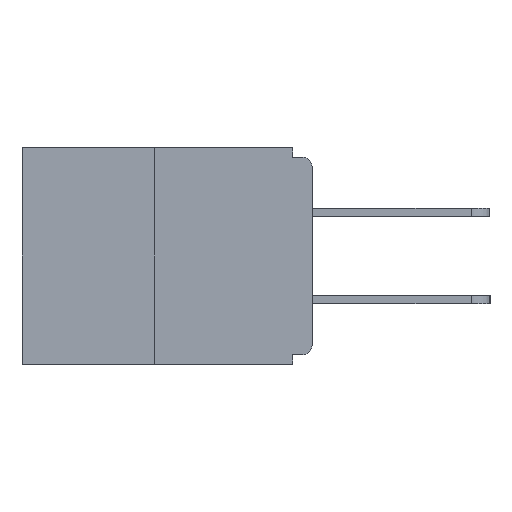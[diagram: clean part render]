
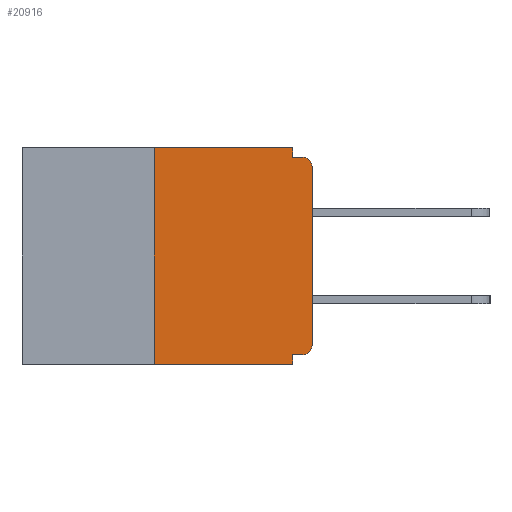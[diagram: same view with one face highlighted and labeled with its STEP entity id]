
A CAD part, left-side view. The second image highlights one B-rep face of the part: STEP entity #20916.
In plain terms, the highlighted planar face has unit normal (-1, 0, 0).
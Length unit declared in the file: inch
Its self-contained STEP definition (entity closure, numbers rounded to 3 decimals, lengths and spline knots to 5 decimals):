
#261 = CARTESIAN_POINT ( 'NONE',  ( 0., 0.015, -0.313 ) ) ;
#347 = EDGE_CURVE ( 'NONE', #24969, #27479, #17518, .T. ) ;
#1140 = VERTEX_POINT ( 'NONE', #24578 ) ;
#1160 = CARTESIAN_POINT ( 'NONE',  ( 0., 0.031, -0.343 ) ) ;
#1166 = VECTOR ( 'NONE', #5473, 39.37008 ) ;
#1633 = PLANE ( 'NONE',  #9875 ) ;
#1690 = DIRECTION ( 'NONE',  ( 0., 0., -1. ) ) ;
#1935 = VECTOR ( 'NONE', #3041, 39.37008 ) ;
#2281 = CARTESIAN_POINT ( 'NONE',  ( 0., 0.46, -0.343 ) ) ;
#2293 = LINE ( 'NONE', #9310, #15512 ) ;
#2387 = VERTEX_POINT ( 'NONE', #28183 ) ;
#2487 = DIRECTION ( 'NONE',  ( 0., 1., 0. ) ) ;
#3041 = DIRECTION ( 'NONE',  ( 0., -1., 0. ) ) ;
#3186 = CARTESIAN_POINT ( 'NONE',  ( 0., 0., -0.015 ) ) ;
#3603 = LINE ( 'NONE', #10343, #4824 ) ;
#3840 = FACE_OUTER_BOUND ( 'NONE', #8987, .T. ) ;
#4049 = AXIS2_PLACEMENT_3D ( 'NONE', #15435, #19617, #1690 ) ;
#4186 = CARTESIAN_POINT ( 'NONE',  ( 0., 0., -0.328 ) ) ;
#4238 = LINE ( 'NONE', #6481, #10053 ) ;
#4304 = CARTESIAN_POINT ( 'NONE',  ( 0., 0.015, -0.015 ) ) ;
#4824 = VECTOR ( 'NONE', #28623, 39.37008 ) ;
#5473 = DIRECTION ( 'NONE',  ( 0., 0., 1. ) ) ;
#5676 = EDGE_CURVE ( 'NONE', #1140, #22539, #7380, .T. ) ;
#6481 = CARTESIAN_POINT ( 'NONE',  ( 0., 0.46, 0. ) ) ;
#7315 = VERTEX_POINT ( 'NONE', #25043 ) ;
#7380 = LINE ( 'NONE', #3186, #1935 ) ;
#8625 = DIRECTION ( 'NONE',  ( 1., 0., 0. ) ) ;
#8987 = EDGE_LOOP ( 'NONE', ( #12906, #17962, #13409, #24241, #19077, #13813, #15092, #17164, #25735, #23451 ) ) ;
#9289 = EDGE_CURVE ( 'NONE', #16557, #9814, #13515, .T. ) ;
#9310 = CARTESIAN_POINT ( 'NONE',  ( 0., 0.031, 0. ) ) ;
#9814 = VERTEX_POINT ( 'NONE', #1160 ) ;
#9875 = AXIS2_PLACEMENT_3D ( 'NONE', #10743, #8625, #29024 ) ;
#9969 = CARTESIAN_POINT ( 'NONE',  ( 0., 0., -0.03 ) ) ;
#10053 = VECTOR ( 'NONE', #18315, 39.37008 ) ;
#10123 = VECTOR ( 'NONE', #28257, 39.37008 ) ;
#10343 = CARTESIAN_POINT ( 'NONE',  ( 0., 0.031, -0.343 ) ) ;
#10743 = CARTESIAN_POINT ( 'NONE',  ( 0., 0.46, 0. ) ) ;
#10927 = EDGE_CURVE ( 'NONE', #22735, #22539, #26048, .T. ) ;
#11486 = LINE ( 'NONE', #16267, #1166 ) ;
#12674 = EDGE_CURVE ( 'NONE', #26373, #2387, #4238, .T. ) ;
#12906 = ORIENTED_EDGE ( 'NONE', *, *, #12674, .F. ) ;
#13409 = ORIENTED_EDGE ( 'NONE', *, *, #9289, .T. ) ;
#13515 = LINE ( 'NONE', #2281, #14667 ) ;
#13813 = ORIENTED_EDGE ( 'NONE', *, *, #25436, .T. ) ;
#14301 = EDGE_CURVE ( 'NONE', #16557, #26373, #28420, .T. ) ;
#14667 = VECTOR ( 'NONE', #18156, 39.37008 ) ;
#15092 = ORIENTED_EDGE ( 'NONE', *, *, #18273, .T. ) ;
#15435 = CARTESIAN_POINT ( 'NONE',  ( 0., 0.015, -0.03 ) ) ;
#15512 = VECTOR ( 'NONE', #18447, 39.37008 ) ;
#16267 = CARTESIAN_POINT ( 'NONE',  ( 0., 0., 0. ) ) ;
#16557 = VERTEX_POINT ( 'NONE', #27753 ) ;
#17164 = ORIENTED_EDGE ( 'NONE', *, *, #10927, .T. ) ;
#17518 = LINE ( 'NONE', #4186, #25430 ) ;
#17962 = ORIENTED_EDGE ( 'NONE', *, *, #14301, .F. ) ;
#18156 = DIRECTION ( 'NONE',  ( 0., -1., 0. ) ) ;
#18273 = EDGE_CURVE ( 'NONE', #7315, #22735, #11486, .T. ) ;
#18315 = DIRECTION ( 'NONE',  ( 0., -1., 0. ) ) ;
#18447 = DIRECTION ( 'NONE',  ( 0., 0., -1. ) ) ;
#18525 = EDGE_CURVE ( 'NONE', #2387, #1140, #2293, .T. ) ;
#19077 = ORIENTED_EDGE ( 'NONE', *, *, #347, .F. ) ;
#19617 = DIRECTION ( 'NONE',  ( -1., 0., 0. ) ) ;
#19966 = CARTESIAN_POINT ( 'NONE',  ( 0., 0.031, -0.328 ) ) ;
#20916 = ADVANCED_FACE ( 'NONE', ( #3840 ), #1633, .F. ) ;
#21118 = AXIS2_PLACEMENT_3D ( 'NONE', #261, #27647, #25412 ) ;
#22539 = VERTEX_POINT ( 'NONE', #4304 ) ;
#22592 = CIRCLE ( 'NONE', #21118, 0.015 ) ;
#22735 = VERTEX_POINT ( 'NONE', #9969 ) ;
#22769 = CARTESIAN_POINT ( 'NONE',  ( 0., 0.015, -0.328 ) ) ;
#23451 = ORIENTED_EDGE ( 'NONE', *, *, #18525, .F. ) ;
#24241 = ORIENTED_EDGE ( 'NONE', *, *, #24746, .F. ) ;
#24578 = CARTESIAN_POINT ( 'NONE',  ( 0., 0.031, -0.015 ) ) ;
#24746 = EDGE_CURVE ( 'NONE', #27479, #9814, #3603, .T. ) ;
#24969 = VERTEX_POINT ( 'NONE', #22769 ) ;
#25043 = CARTESIAN_POINT ( 'NONE',  ( 0., 0., -0.313 ) ) ;
#25412 = DIRECTION ( 'NONE',  ( 0., 0., -1. ) ) ;
#25430 = VECTOR ( 'NONE', #2487, 39.37008 ) ;
#25436 = EDGE_CURVE ( 'NONE', #24969, #7315, #22592, .T. ) ;
#25735 = ORIENTED_EDGE ( 'NONE', *, *, #5676, .F. ) ;
#26048 = CIRCLE ( 'NONE', #4049, 0.015 ) ;
#26373 = VERTEX_POINT ( 'NONE', #27892 ) ;
#27479 = VERTEX_POINT ( 'NONE', #19966 ) ;
#27647 = DIRECTION ( 'NONE',  ( -1., 0., 0. ) ) ;
#27753 = CARTESIAN_POINT ( 'NONE',  ( 0., 0.25, -0.343 ) ) ;
#27892 = CARTESIAN_POINT ( 'NONE',  ( 0., 0.25, 0. ) ) ;
#28183 = CARTESIAN_POINT ( 'NONE',  ( 0., 0.031, 0. ) ) ;
#28257 = DIRECTION ( 'NONE',  ( 0., 0., 1. ) ) ;
#28420 = LINE ( 'NONE', #28572, #10123 ) ;
#28572 = CARTESIAN_POINT ( 'NONE',  ( 0., 0.25, 0. ) ) ;
#28623 = DIRECTION ( 'NONE',  ( 0., 0., -1. ) ) ;
#29024 = DIRECTION ( 'NONE',  ( 0., 0., -1. ) ) ;
